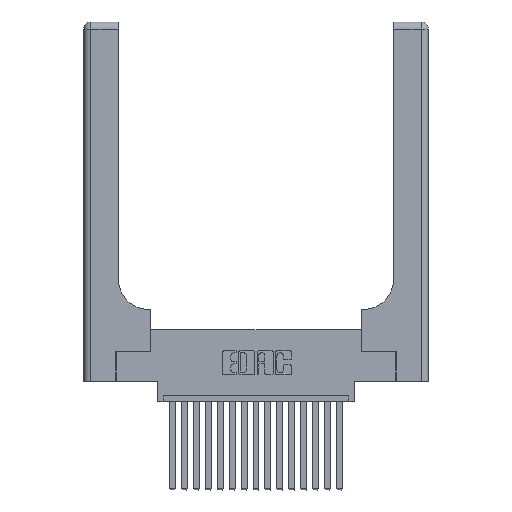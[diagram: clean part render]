
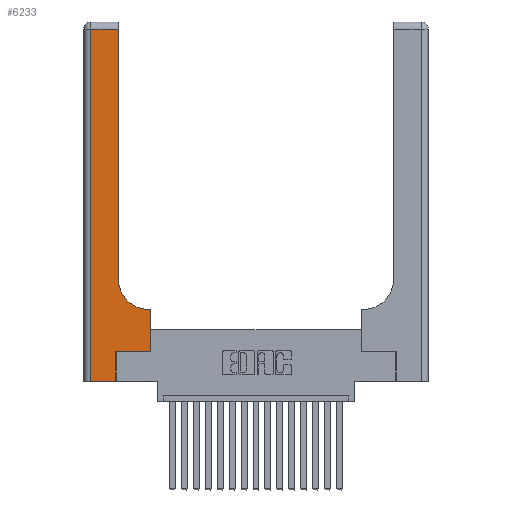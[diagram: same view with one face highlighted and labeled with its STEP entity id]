
A CAD part, top view. The second image highlights one B-rep face of the part: STEP entity #6233.
In plain terms, the highlighted planar face has unit normal (0, 0, 1).
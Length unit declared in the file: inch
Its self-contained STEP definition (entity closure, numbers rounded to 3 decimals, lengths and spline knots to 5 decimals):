
#49 = FACE_OUTER_BOUND ( 'NONE', #4266, .T. ) ;
#478 = CARTESIAN_POINT ( 'NONE',  ( 0.5415, 0.85, 0.37 ) ) ;
#487 = VECTOR ( 'NONE', #12022, 39.37008 ) ;
#513 = LINE ( 'NONE', #546, #17937 ) ;
#546 = CARTESIAN_POINT ( 'NONE',  ( 0., 0., 0.37 ) ) ;
#978 = ORIENTED_EDGE ( 'NONE', *, *, #3953, .T. ) ;
#1089 = DIRECTION ( 'NONE',  ( 1., 0., 0. ) ) ;
#1160 = ORIENTED_EDGE ( 'NONE', *, *, #2605, .T. ) ;
#1362 = VERTEX_POINT ( 'NONE', #8278 ) ;
#1498 = VERTEX_POINT ( 'NONE', #2453 ) ;
#1850 = CARTESIAN_POINT ( 'NONE',  ( 0.06, 0., 0.37 ) ) ;
#1887 = LINE ( 'NONE', #13181, #9895 ) ;
#2098 = DIRECTION ( 'NONE',  ( 1., 0., 0. ) ) ;
#2116 = CARTESIAN_POINT ( 'NONE',  ( 0.269, 0.25, 0.37 ) ) ;
#2400 = ORIENTED_EDGE ( 'NONE', *, *, #3642, .T. ) ;
#2402 = CARTESIAN_POINT ( 'NONE',  ( 0.2915, 2.94, 0.37 ) ) ;
#2453 = CARTESIAN_POINT ( 'NONE',  ( 0.2915, 0.85, 0.37 ) ) ;
#2605 = EDGE_CURVE ( 'NONE', #17018, #1498, #9437, .T. ) ;
#2715 = CARTESIAN_POINT ( 'NONE',  ( 0., 2.94, 0.37 ) ) ;
#2742 = AXIS2_PLACEMENT_3D ( 'NONE', #478, #13256, #1089 ) ;
#2925 = ORIENTED_EDGE ( 'NONE', *, *, #13435, .T. ) ;
#3642 = EDGE_CURVE ( 'NONE', #14820, #12619, #10336, .T. ) ;
#3953 = EDGE_CURVE ( 'NONE', #1362, #13774, #4305, .T. ) ;
#4012 = VECTOR ( 'NONE', #7033, 39.37008 ) ;
#4152 = DIRECTION ( 'NONE',  ( 0., 1., 0. ) ) ;
#4266 = EDGE_LOOP ( 'NONE', ( #10203, #2400, #16663, #16102, #19408, #2925, #978, #13592, #1160 ) ) ;
#4305 = LINE ( 'NONE', #17920, #16857 ) ;
#4815 = VERTEX_POINT ( 'NONE', #8197 ) ;
#4963 = EDGE_CURVE ( 'NONE', #12619, #13375, #5944, .T. ) ;
#5944 = LINE ( 'NONE', #13183, #4012 ) ;
#5960 = EDGE_CURVE ( 'NONE', #4815, #16973, #14855, .T. ) ;
#5984 = CARTESIAN_POINT ( 'NONE',  ( 0., 3., 0.37 ) ) ;
#6233 = ADVANCED_FACE ( 'NONE', ( #49 ), #13685, .F. ) ;
#7033 = DIRECTION ( 'NONE',  ( 0., -1., 0. ) ) ;
#7052 = CARTESIAN_POINT ( 'NONE',  ( 0.269, 0.25, 0.37 ) ) ;
#7383 = DIRECTION ( 'NONE',  ( -1., 0., 0. ) ) ;
#7471 = CARTESIAN_POINT ( 'NONE',  ( 0.2915, 0.6, 0.37 ) ) ;
#7592 = CARTESIAN_POINT ( 'NONE',  ( 0.5585, 0.6, 0.37 ) ) ;
#8137 = EDGE_CURVE ( 'NONE', #13375, #4815, #513, .T. ) ;
#8197 = CARTESIAN_POINT ( 'NONE',  ( 0.269, 0., 0.37 ) ) ;
#8278 = CARTESIAN_POINT ( 'NONE',  ( 0.5585, 0.25, 0.37 ) ) ;
#8430 = CARTESIAN_POINT ( 'NONE',  ( 0.269, 0., 0.37 ) ) ;
#8558 = DIRECTION ( 'NONE',  ( 1., 0., 0. ) ) ;
#8900 = DIRECTION ( 'NONE',  ( 0., 0., -1. ) ) ;
#9380 = VECTOR ( 'NONE', #7383, 39.37008 ) ;
#9437 = CIRCLE ( 'NONE', #2742, 0.25 ) ;
#9895 = VECTOR ( 'NONE', #16239, 39.37008 ) ;
#9925 = EDGE_CURVE ( 'NONE', #1498, #14820, #1887, .T. ) ;
#10203 = ORIENTED_EDGE ( 'NONE', *, *, #9925, .T. ) ;
#10336 = LINE ( 'NONE', #2715, #9380 ) ;
#11112 = CARTESIAN_POINT ( 'NONE',  ( 0.5415, 0.6, 0.37 ) ) ;
#11633 = LINE ( 'NONE', #7471, #487 ) ;
#12022 = DIRECTION ( 'NONE',  ( -1., 0., 0. ) ) ;
#12619 = VERTEX_POINT ( 'NONE', #19853 ) ;
#12959 = DIRECTION ( 'NONE',  ( 0., 1., 0. ) ) ;
#13181 = CARTESIAN_POINT ( 'NONE',  ( 0.2915, 3., 0.37 ) ) ;
#13183 = CARTESIAN_POINT ( 'NONE',  ( 0.06, 3., 0.37 ) ) ;
#13198 = VECTOR ( 'NONE', #8558, 39.37008 ) ;
#13256 = DIRECTION ( 'NONE',  ( 0., 0., -1. ) ) ;
#13375 = VERTEX_POINT ( 'NONE', #1850 ) ;
#13392 = VECTOR ( 'NONE', #12959, 39.37008 ) ;
#13435 = EDGE_CURVE ( 'NONE', #16973, #1362, #16850, .T. ) ;
#13592 = ORIENTED_EDGE ( 'NONE', *, *, #18351, .T. ) ;
#13685 = PLANE ( 'NONE',  #17155 ) ;
#13774 = VERTEX_POINT ( 'NONE', #7592 ) ;
#14820 = VERTEX_POINT ( 'NONE', #2402 ) ;
#14855 = LINE ( 'NONE', #8430, #13392 ) ;
#16102 = ORIENTED_EDGE ( 'NONE', *, *, #8137, .T. ) ;
#16239 = DIRECTION ( 'NONE',  ( 0., 1., 0. ) ) ;
#16663 = ORIENTED_EDGE ( 'NONE', *, *, #4963, .T. ) ;
#16850 = LINE ( 'NONE', #7052, #13198 ) ;
#16857 = VECTOR ( 'NONE', #4152, 39.37008 ) ;
#16973 = VERTEX_POINT ( 'NONE', #2116 ) ;
#17018 = VERTEX_POINT ( 'NONE', #11112 ) ;
#17155 = AXIS2_PLACEMENT_3D ( 'NONE', #5984, #8900, #18214 ) ;
#17920 = CARTESIAN_POINT ( 'NONE',  ( 0.5585, 0.25, 0.37 ) ) ;
#17937 = VECTOR ( 'NONE', #2098, 39.37008 ) ;
#18214 = DIRECTION ( 'NONE',  ( -1., 0., 0. ) ) ;
#18351 = EDGE_CURVE ( 'NONE', #13774, #17018, #11633, .T. ) ;
#19408 = ORIENTED_EDGE ( 'NONE', *, *, #5960, .T. ) ;
#19853 = CARTESIAN_POINT ( 'NONE',  ( 0.06, 2.94, 0.37 ) ) ;
